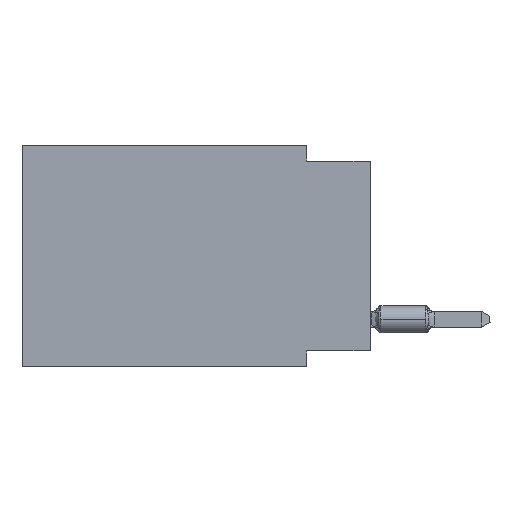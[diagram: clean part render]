
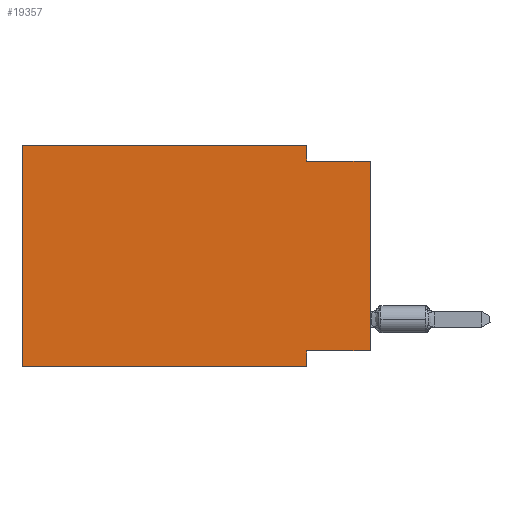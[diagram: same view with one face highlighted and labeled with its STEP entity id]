
A CAD part, left-side view. The second image highlights one B-rep face of the part: STEP entity #19357.
In plain terms, the highlighted planar face has unit normal (-1, 0, 0).
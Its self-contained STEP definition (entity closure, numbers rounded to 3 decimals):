
#432 = CARTESIAN_POINT ( 'NONE',  ( 0., 13.97, -8.89 ) ) ;
#472 = ORIENTED_EDGE ( 'NONE', *, *, #11686, .F. ) ;
#492 = DIRECTION ( 'NONE',  ( 0., 0., -1. ) ) ;
#662 = EDGE_CURVE ( 'NONE', #7303, #16284, #20850, .T. ) ;
#1059 = DIRECTION ( 'NONE',  ( 0., -1., 0. ) ) ;
#1421 = ORIENTED_EDGE ( 'NONE', *, *, #5219, .T. ) ;
#1658 = DIRECTION ( 'NONE',  ( 0., 0., 1. ) ) ;
#1697 = CARTESIAN_POINT ( 'NONE',  ( 0., 13.97, -8.89 ) ) ;
#2057 = VERTEX_POINT ( 'NONE', #19673 ) ;
#3165 = ORIENTED_EDGE ( 'NONE', *, *, #11017, .F. ) ;
#3434 = LINE ( 'NONE', #13176, #17936 ) ;
#3499 = EDGE_CURVE ( 'NONE', #7303, #16857, #14289, .T. ) ;
#4238 = DIRECTION ( 'NONE',  ( 1., 0., 0. ) ) ;
#4444 = PLANE ( 'NONE',  #10620 ) ;
#4607 = ORIENTED_EDGE ( 'NONE', *, *, #10919, .F. ) ;
#4901 = VERTEX_POINT ( 'NONE', #10332 ) ;
#5219 = EDGE_CURVE ( 'NONE', #4901, #2057, #16529, .T. ) ;
#5398 = LINE ( 'NONE', #6899, #19587 ) ;
#5832 = FACE_OUTER_BOUND ( 'NONE', #14161, .T. ) ;
#6255 = VECTOR ( 'NONE', #1059, 1000. ) ;
#6409 = ORIENTED_EDGE ( 'NONE', *, *, #7261, .F. ) ;
#6435 = EDGE_CURVE ( 'NONE', #16857, #12404, #15518, .T. ) ;
#6899 = CARTESIAN_POINT ( 'NONE',  ( 0., 2.54, 0. ) ) ;
#7017 = ORIENTED_EDGE ( 'NONE', *, *, #6435, .F. ) ;
#7219 = CARTESIAN_POINT ( 'NONE',  ( 0., 0., -0.635 ) ) ;
#7261 = EDGE_CURVE ( 'NONE', #4901, #10024, #15114, .T. ) ;
#7303 = VERTEX_POINT ( 'NONE', #432 ) ;
#7416 = ORIENTED_EDGE ( 'NONE', *, *, #3499, .F. ) ;
#8337 = DIRECTION ( 'NONE',  ( 0., 1., 0. ) ) ;
#8746 = CARTESIAN_POINT ( 'NONE',  ( 0., 13.97, 0. ) ) ;
#10024 = VERTEX_POINT ( 'NONE', #13946 ) ;
#10332 = CARTESIAN_POINT ( 'NONE',  ( 0., 0., -8.255 ) ) ;
#10620 = AXIS2_PLACEMENT_3D ( 'NONE', #20702, #4238, #12481 ) ;
#10648 = DIRECTION ( 'NONE',  ( 0., 0., 1. ) ) ;
#10919 = EDGE_CURVE ( 'NONE', #12404, #11908, #5398, .T. ) ;
#11017 = EDGE_CURVE ( 'NONE', #11908, #2057, #11841, .T. ) ;
#11050 = VECTOR ( 'NONE', #18712, 1000. ) ;
#11614 = CARTESIAN_POINT ( 'NONE',  ( 0., 2.54, -8.89 ) ) ;
#11686 = EDGE_CURVE ( 'NONE', #10024, #16284, #3434, .T. ) ;
#11784 = DIRECTION ( 'NONE',  ( 0., 0., -1. ) ) ;
#11841 = LINE ( 'NONE', #7219, #11050 ) ;
#11908 = VERTEX_POINT ( 'NONE', #20840 ) ;
#12047 = VECTOR ( 'NONE', #1658, 1000. ) ;
#12404 = VERTEX_POINT ( 'NONE', #20706 ) ;
#12481 = DIRECTION ( 'NONE',  ( 0., 0., -1. ) ) ;
#13176 = CARTESIAN_POINT ( 'NONE',  ( 0., 2.54, -8.89 ) ) ;
#13281 = CARTESIAN_POINT ( 'NONE',  ( 0., 0., -8.255 ) ) ;
#13946 = CARTESIAN_POINT ( 'NONE',  ( 0., 2.54, -8.255 ) ) ;
#14161 = EDGE_LOOP ( 'NONE', ( #1421, #3165, #4607, #7017, #7416, #19775, #472, #6409 ) ) ;
#14289 = LINE ( 'NONE', #20905, #17150 ) ;
#14385 = CARTESIAN_POINT ( 'NONE',  ( 0., 13.97, 0. ) ) ;
#14949 = VECTOR ( 'NONE', #19461, 1000. ) ;
#15114 = LINE ( 'NONE', #13281, #20632 ) ;
#15518 = LINE ( 'NONE', #8746, #6255 ) ;
#16284 = VERTEX_POINT ( 'NONE', #11614 ) ;
#16529 = LINE ( 'NONE', #17829, #12047 ) ;
#16857 = VERTEX_POINT ( 'NONE', #14385 ) ;
#17150 = VECTOR ( 'NONE', #10648, 1000. ) ;
#17829 = CARTESIAN_POINT ( 'NONE',  ( 0., 0., 0. ) ) ;
#17936 = VECTOR ( 'NONE', #11784, 1000. ) ;
#18712 = DIRECTION ( 'NONE',  ( 0., -1., 0. ) ) ;
#19357 = ADVANCED_FACE ( 'NONE', ( #5832 ), #4444, .F. ) ;
#19461 = DIRECTION ( 'NONE',  ( 0., -1., 0. ) ) ;
#19587 = VECTOR ( 'NONE', #492, 1000. ) ;
#19673 = CARTESIAN_POINT ( 'NONE',  ( 0., 0., -0.635 ) ) ;
#19775 = ORIENTED_EDGE ( 'NONE', *, *, #662, .T. ) ;
#20632 = VECTOR ( 'NONE', #8337, 1000. ) ;
#20702 = CARTESIAN_POINT ( 'NONE',  ( 0., 13.97, 0. ) ) ;
#20706 = CARTESIAN_POINT ( 'NONE',  ( 0., 2.54, 0. ) ) ;
#20840 = CARTESIAN_POINT ( 'NONE',  ( 0., 2.54, -0.635 ) ) ;
#20850 = LINE ( 'NONE', #1697, #14949 ) ;
#20905 = CARTESIAN_POINT ( 'NONE',  ( 0., 13.97, 0. ) ) ;
